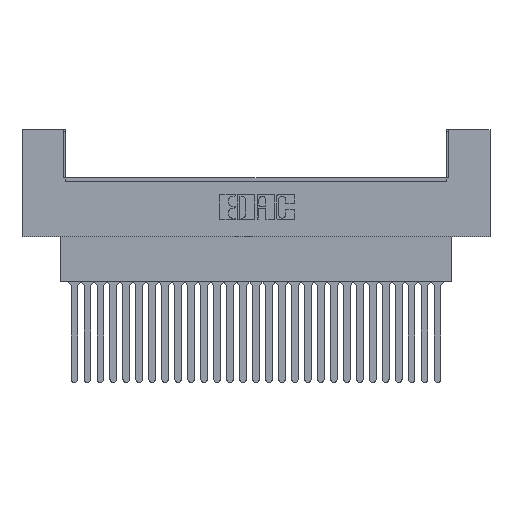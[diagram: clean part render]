
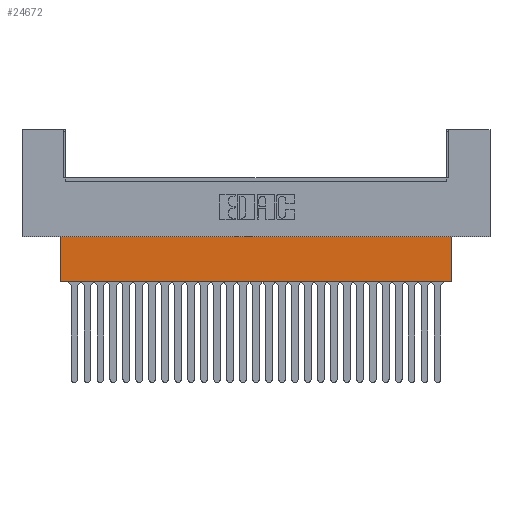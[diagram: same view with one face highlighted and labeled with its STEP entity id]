
A CAD part, top view. The second image highlights one B-rep face of the part: STEP entity #24672.
In plain terms, the highlighted planar face has unit normal (0, 0, 1).
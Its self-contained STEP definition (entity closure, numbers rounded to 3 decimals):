
#2814 = LINE ( 'NONE', #23656, #30113 ) ;
#3418 = CARTESIAN_POINT ( 'NONE',  ( 91.592, 0., -3.962 ) ) ;
#5317 = VECTOR ( 'NONE', #32880, 1000. ) ;
#7259 = CARTESIAN_POINT ( 'NONE',  ( 84.125, -8.814, -3.962 ) ) ;
#8452 = ORIENTED_EDGE ( 'NONE', *, *, #25830, .T. ) ;
#9961 = DIRECTION ( 'NONE',  ( 0., 0., -1. ) ) ;
#10189 = PLANE ( 'NONE',  #32674 ) ;
#12259 = VECTOR ( 'NONE', #27081, 1000. ) ;
#12669 = DIRECTION ( 'NONE',  ( -1., 0., 0. ) ) ;
#13319 = CARTESIAN_POINT ( 'NONE',  ( 84.125, 0., -3.962 ) ) ;
#14768 = VECTOR ( 'NONE', #25247, 1000. ) ;
#15458 = CARTESIAN_POINT ( 'NONE',  ( 91.592, 0., -3.962 ) ) ;
#15928 = DIRECTION ( 'NONE',  ( 0., 1., 0. ) ) ;
#18932 = VERTEX_POINT ( 'NONE', #21699 ) ;
#19307 = VERTEX_POINT ( 'NONE', #7259 ) ;
#21699 = CARTESIAN_POINT ( 'NONE',  ( 7.468, -8.814, -3.962 ) ) ;
#23656 = CARTESIAN_POINT ( 'NONE',  ( 91.592, -8.814, -3.962 ) ) ;
#23674 = EDGE_CURVE ( 'NONE', #18932, #32342, #31445, .T. ) ;
#23751 = LINE ( 'NONE', #3418, #14768 ) ;
#23884 = CARTESIAN_POINT ( 'NONE',  ( 7.468, -8.814, -3.962 ) ) ;
#24573 = ORIENTED_EDGE ( 'NONE', *, *, #23674, .F. ) ;
#24672 = ADVANCED_FACE ( 'NONE', ( #25002 ), #10189, .F. ) ;
#25002 = FACE_OUTER_BOUND ( 'NONE', #31010, .T. ) ;
#25133 = CARTESIAN_POINT ( 'NONE',  ( 84.125, -8.814, -3.962 ) ) ;
#25247 = DIRECTION ( 'NONE',  ( -1., 0., 0. ) ) ;
#25542 = ORIENTED_EDGE ( 'NONE', *, *, #26410, .F. ) ;
#25762 = LINE ( 'NONE', #25133, #5317 ) ;
#25830 = EDGE_CURVE ( 'NONE', #32067, #32342, #23751, .T. ) ;
#26410 = EDGE_CURVE ( 'NONE', #19307, #18932, #2814, .T. ) ;
#27081 = DIRECTION ( 'NONE',  ( 0., 1., 0. ) ) ;
#30113 = VECTOR ( 'NONE', #12669, 1000. ) ;
#31010 = EDGE_LOOP ( 'NONE', ( #25542, #33941, #8452, #24573 ) ) ;
#31172 = CARTESIAN_POINT ( 'NONE',  ( 7.468, 0., -3.962 ) ) ;
#31445 = LINE ( 'NONE', #23884, #12259 ) ;
#32067 = VERTEX_POINT ( 'NONE', #13319 ) ;
#32342 = VERTEX_POINT ( 'NONE', #31172 ) ;
#32674 = AXIS2_PLACEMENT_3D ( 'NONE', #15458, #9961, #15928 ) ;
#32880 = DIRECTION ( 'NONE',  ( 0., -1., 0. ) ) ;
#33941 = ORIENTED_EDGE ( 'NONE', *, *, #34722, .F. ) ;
#34722 = EDGE_CURVE ( 'NONE', #32067, #19307, #25762, .T. ) ;
